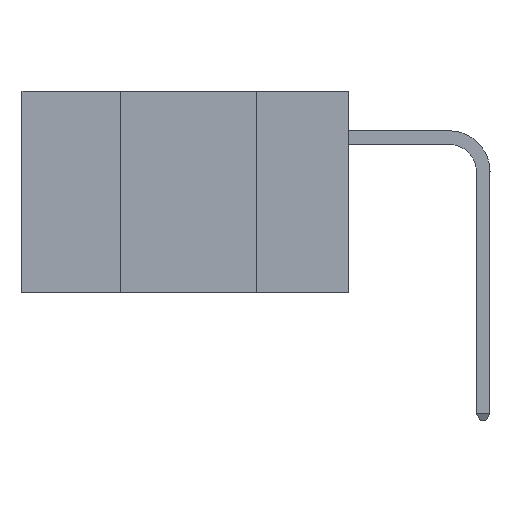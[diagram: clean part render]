
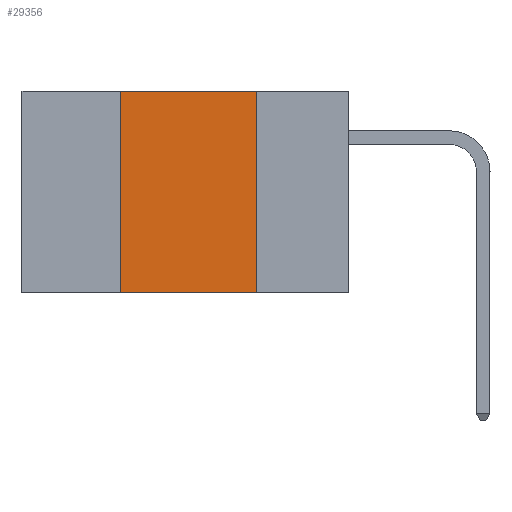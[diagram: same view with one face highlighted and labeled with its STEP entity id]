
A CAD part, left-side view. The second image highlights one B-rep face of the part: STEP entity #29356.
In plain terms, the highlighted planar face has unit normal (-1, 0, 0).
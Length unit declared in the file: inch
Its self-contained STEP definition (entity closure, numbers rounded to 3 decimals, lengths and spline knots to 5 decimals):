
#1942 = LINE ( 'NONE', #37753, #44269 ) ;
#2736 = LINE ( 'NONE', #34803, #35746 ) ;
#3208 = FACE_OUTER_BOUND ( 'NONE', #29056, .T. ) ;
#4806 = VERTEX_POINT ( 'NONE', #35816 ) ;
#6786 = DIRECTION ( 'NONE',  ( 0., 0., -1. ) ) ;
#6997 = ORIENTED_EDGE ( 'NONE', *, *, #33782, .F. ) ;
#10524 = CARTESIAN_POINT ( 'NONE',  ( 0., 0.17, 0. ) ) ;
#11613 = ORIENTED_EDGE ( 'NONE', *, *, #48605, .F. ) ;
#11989 = DIRECTION ( 'NONE',  ( 0., -1., 0. ) ) ;
#13589 = CARTESIAN_POINT ( 'NONE',  ( 0., 0.6, 0. ) ) ;
#13629 = EDGE_CURVE ( 'NONE', #4806, #45167, #1942, .T. ) ;
#14053 = ORIENTED_EDGE ( 'NONE', *, *, #13629, .F. ) ;
#17847 = VECTOR ( 'NONE', #11989, 39.37008 ) ;
#18355 = LINE ( 'NONE', #13589, #50097 ) ;
#20998 = VERTEX_POINT ( 'NONE', #10524 ) ;
#21591 = DIRECTION ( 'NONE',  ( 0., -1., 0. ) ) ;
#21759 = DIRECTION ( 'NONE',  ( 0., 0., -1. ) ) ;
#26749 = EDGE_CURVE ( 'NONE', #4806, #29164, #43389, .T. ) ;
#27529 = CARTESIAN_POINT ( 'NONE',  ( 0., 0.42, 0. ) ) ;
#27804 = CARTESIAN_POINT ( 'NONE',  ( 0., 0.6, -0.37 ) ) ;
#29056 = EDGE_LOOP ( 'NONE', ( #6997, #11613, #14053, #46728 ) ) ;
#29164 = VERTEX_POINT ( 'NONE', #31920 ) ;
#29356 = ADVANCED_FACE ( 'NONE', ( #3208 ), #38140, .F. ) ;
#31490 = AXIS2_PLACEMENT_3D ( 'NONE', #45593, #37968, #21759 ) ;
#31920 = CARTESIAN_POINT ( 'NONE',  ( 0., 0.17, -0.37 ) ) ;
#33782 = EDGE_CURVE ( 'NONE', #20998, #29164, #2736, .T. ) ;
#34803 = CARTESIAN_POINT ( 'NONE',  ( 0., 0.17, 0. ) ) ;
#35746 = VECTOR ( 'NONE', #6786, 39.37008 ) ;
#35816 = CARTESIAN_POINT ( 'NONE',  ( 0., 0.42, -0.37 ) ) ;
#37753 = CARTESIAN_POINT ( 'NONE',  ( 0., 0.42, 0. ) ) ;
#37968 = DIRECTION ( 'NONE',  ( 1., 0., 0. ) ) ;
#38086 = DIRECTION ( 'NONE',  ( 0., 0., 1. ) ) ;
#38140 = PLANE ( 'NONE',  #31490 ) ;
#43389 = LINE ( 'NONE', #27804, #17847 ) ;
#44269 = VECTOR ( 'NONE', #38086, 39.37008 ) ;
#45167 = VERTEX_POINT ( 'NONE', #27529 ) ;
#45593 = CARTESIAN_POINT ( 'NONE',  ( 0., 0.6, 0. ) ) ;
#46728 = ORIENTED_EDGE ( 'NONE', *, *, #26749, .T. ) ;
#48605 = EDGE_CURVE ( 'NONE', #45167, #20998, #18355, .T. ) ;
#50097 = VECTOR ( 'NONE', #21591, 39.37008 ) ;
